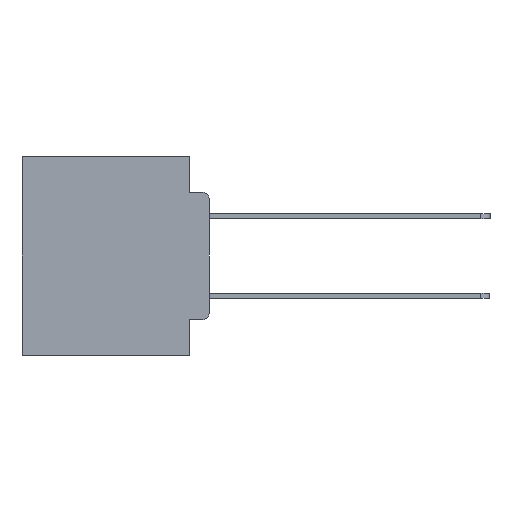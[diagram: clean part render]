
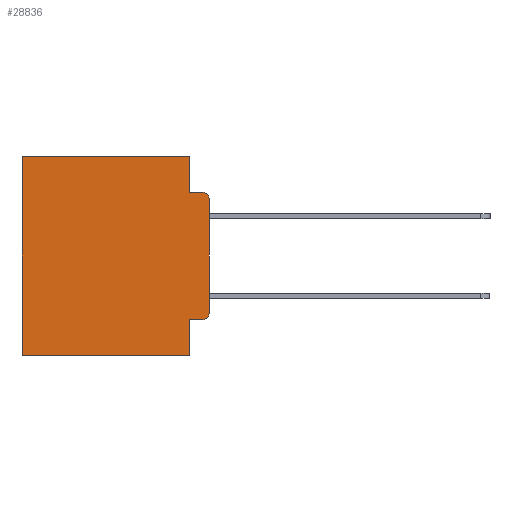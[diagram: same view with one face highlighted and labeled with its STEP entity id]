
A CAD part, left-side view. The second image highlights one B-rep face of the part: STEP entity #28836.
In plain terms, the highlighted planar face has unit normal (-1, 0, 0).
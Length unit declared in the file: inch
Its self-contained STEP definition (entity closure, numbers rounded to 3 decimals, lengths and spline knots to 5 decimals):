
#1017 = AXIS2_PLACEMENT_3D ( 'NONE', #26213, #28427, #14847 ) ;
#1157 = VECTOR ( 'NONE', #27773, 39.37008 ) ;
#1422 = EDGE_CURVE ( 'NONE', #22166, #5241, #7684, .T. ) ;
#1442 = VERTEX_POINT ( 'NONE', #7049 ) ;
#1607 = AXIS2_PLACEMENT_3D ( 'NONE', #9764, #25755, #12074 ) ;
#1953 = CARTESIAN_POINT ( 'NONE',  ( 0.298, 0.051, -0.4115 ) ) ;
#1996 = EDGE_CURVE ( 'NONE', #24887, #21446, #24490, .T. ) ;
#2573 = VECTOR ( 'NONE', #6741, 39.37008 ) ;
#3058 = VERTEX_POINT ( 'NONE', #9398 ) ;
#3187 = EDGE_CURVE ( 'NONE', #4811, #3058, #28604, .T. ) ;
#3188 = DIRECTION ( 'NONE',  ( 0., 0., -1. ) ) ;
#3695 = ORIENTED_EDGE ( 'NONE', *, *, #29620, .T. ) ;
#4288 = VECTOR ( 'NONE', #23474, 39.37008 ) ;
#4401 = CARTESIAN_POINT ( 'NONE',  ( 0.298, 0.051, -0.0885 ) ) ;
#4418 = EDGE_CURVE ( 'NONE', #21446, #1442, #10460, .T. ) ;
#4527 = VERTEX_POINT ( 'NONE', #26203 ) ;
#4811 = VERTEX_POINT ( 'NONE', #14468 ) ;
#5067 = DIRECTION ( 'NONE',  ( 0., 0., -1. ) ) ;
#5241 = VERTEX_POINT ( 'NONE', #8640 ) ;
#5537 = ORIENTED_EDGE ( 'NONE', *, *, #9369, .F. ) ;
#5554 = VECTOR ( 'NONE', #28811, 39.37008 ) ;
#5621 = VERTEX_POINT ( 'NONE', #17400 ) ;
#6741 = DIRECTION ( 'NONE',  ( 0., -1., 0. ) ) ;
#6964 = ORIENTED_EDGE ( 'NONE', *, *, #18777, .T. ) ;
#7049 = CARTESIAN_POINT ( 'NONE',  ( 0.298, 0.473, -0.5 ) ) ;
#7684 = CIRCLE ( 'NONE', #23665, 0.02 ) ;
#7696 = EDGE_CURVE ( 'NONE', #23919, #4527, #25605, .T. ) ;
#7739 = CARTESIAN_POINT ( 'NONE',  ( 0.298, 0.051, -0.0885 ) ) ;
#8499 = LINE ( 'NONE', #21609, #26019 ) ;
#8640 = CARTESIAN_POINT ( 'NONE',  ( 0.298, 0., -0.3915 ) ) ;
#9369 = EDGE_CURVE ( 'NONE', #4811, #23919, #13530, .T. ) ;
#9398 = CARTESIAN_POINT ( 'NONE',  ( 0.298, 0.473, 0. ) ) ;
#9524 = CARTESIAN_POINT ( 'NONE',  ( 0.298, 0.051, 0. ) ) ;
#9764 = CARTESIAN_POINT ( 'NONE',  ( 0.298, 0.02, -0.1085 ) ) ;
#10460 = LINE ( 'NONE', #23579, #4288 ) ;
#10949 = CIRCLE ( 'NONE', #1607, 0.02 ) ;
#10968 = ORIENTED_EDGE ( 'NONE', *, *, #17172, .F. ) ;
#11329 = ORIENTED_EDGE ( 'NONE', *, *, #1422, .T. ) ;
#11708 = LINE ( 'NONE', #12937, #5554 ) ;
#12074 = DIRECTION ( 'NONE',  ( 0., 0., -1. ) ) ;
#12937 = CARTESIAN_POINT ( 'NONE',  ( 0.298, 0.051, -0.4115 ) ) ;
#12990 = EDGE_LOOP ( 'NONE', ( #10968, #6964, #13113, #5537, #14535, #27349, #19597, #16696, #3695, #11329 ) ) ;
#13068 = VECTOR ( 'NONE', #20034, 39.37008 ) ;
#13113 = ORIENTED_EDGE ( 'NONE', *, *, #7696, .F. ) ;
#13216 = LINE ( 'NONE', #21126, #19301 ) ;
#13530 = LINE ( 'NONE', #14165, #1157 ) ;
#14165 = CARTESIAN_POINT ( 'NONE',  ( 0.298, 0.051, 0. ) ) ;
#14468 = CARTESIAN_POINT ( 'NONE',  ( 0.298, 0.051, 0. ) ) ;
#14535 = ORIENTED_EDGE ( 'NONE', *, *, #3187, .T. ) ;
#14847 = DIRECTION ( 'NONE',  ( 0., 0., -1. ) ) ;
#15003 = FACE_OUTER_BOUND ( 'NONE', #12990, .T. ) ;
#16501 = DIRECTION ( 'NONE',  ( -1., 0., 0. ) ) ;
#16579 = DIRECTION ( 'NONE',  ( 0., 0., -1. ) ) ;
#16696 = ORIENTED_EDGE ( 'NONE', *, *, #1996, .F. ) ;
#17172 = EDGE_CURVE ( 'NONE', #5621, #5241, #8499, .T. ) ;
#17400 = CARTESIAN_POINT ( 'NONE',  ( 0.298, 0., -0.1085 ) ) ;
#17881 = DIRECTION ( 'NONE',  ( 0., 1., 0. ) ) ;
#18215 = CARTESIAN_POINT ( 'NONE',  ( 0.298, 0., 0. ) ) ;
#18777 = EDGE_CURVE ( 'NONE', #5621, #4527, #10949, .T. ) ;
#19301 = VECTOR ( 'NONE', #5067, 39.37008 ) ;
#19597 = ORIENTED_EDGE ( 'NONE', *, *, #4418, .F. ) ;
#20034 = DIRECTION ( 'NONE',  ( 0., 0., -1. ) ) ;
#21126 = CARTESIAN_POINT ( 'NONE',  ( 0.298, 0.473, 0. ) ) ;
#21193 = VECTOR ( 'NONE', #17881, 39.37008 ) ;
#21446 = VERTEX_POINT ( 'NONE', #24470 ) ;
#21609 = CARTESIAN_POINT ( 'NONE',  ( 0.298, 0., 0. ) ) ;
#22166 = VERTEX_POINT ( 'NONE', #27091 ) ;
#22858 = CARTESIAN_POINT ( 'NONE',  ( 0.298, 0.02, -0.3915 ) ) ;
#23474 = DIRECTION ( 'NONE',  ( 0., 1., 0. ) ) ;
#23579 = CARTESIAN_POINT ( 'NONE',  ( 0.298, 0., -0.5 ) ) ;
#23665 = AXIS2_PLACEMENT_3D ( 'NONE', #22858, #16501, #16579 ) ;
#23913 = PLANE ( 'NONE',  #1017 ) ;
#23919 = VERTEX_POINT ( 'NONE', #7739 ) ;
#24470 = CARTESIAN_POINT ( 'NONE',  ( 0.298, 0.051, -0.5 ) ) ;
#24490 = LINE ( 'NONE', #9524, #13068 ) ;
#24887 = VERTEX_POINT ( 'NONE', #1953 ) ;
#25605 = LINE ( 'NONE', #4401, #2573 ) ;
#25755 = DIRECTION ( 'NONE',  ( -1., 0., 0. ) ) ;
#26019 = VECTOR ( 'NONE', #3188, 39.37008 ) ;
#26203 = CARTESIAN_POINT ( 'NONE',  ( 0.298, 0.02, -0.0885 ) ) ;
#26213 = CARTESIAN_POINT ( 'NONE',  ( 0.298, 0., 0. ) ) ;
#27091 = CARTESIAN_POINT ( 'NONE',  ( 0.298, 0.02, -0.4115 ) ) ;
#27349 = ORIENTED_EDGE ( 'NONE', *, *, #28681, .T. ) ;
#27773 = DIRECTION ( 'NONE',  ( 0., 0., -1. ) ) ;
#28427 = DIRECTION ( 'NONE',  ( 1., 0., 0. ) ) ;
#28604 = LINE ( 'NONE', #18215, #21193 ) ;
#28681 = EDGE_CURVE ( 'NONE', #3058, #1442, #13216, .T. ) ;
#28811 = DIRECTION ( 'NONE',  ( 0., -1., 0. ) ) ;
#28836 = ADVANCED_FACE ( 'NONE', ( #15003 ), #23913, .F. ) ;
#29620 = EDGE_CURVE ( 'NONE', #24887, #22166, #11708, .T. ) ;
